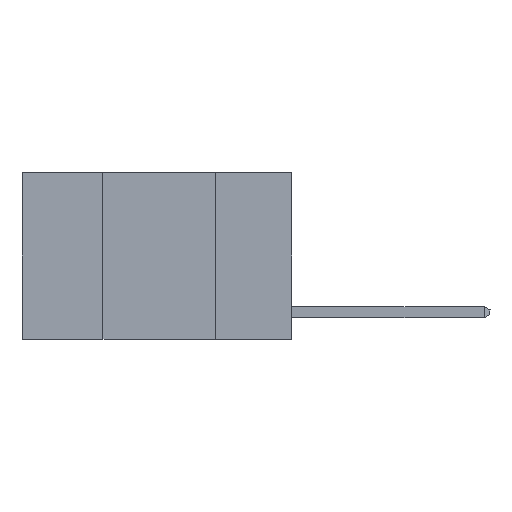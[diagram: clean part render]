
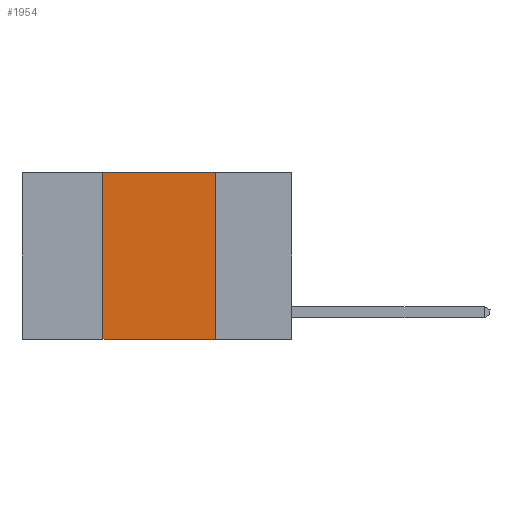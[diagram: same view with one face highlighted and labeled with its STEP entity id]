
A CAD part, left-side view. The second image highlights one B-rep face of the part: STEP entity #1954.
In plain terms, the highlighted planar face has unit normal (-1, 0, 0).
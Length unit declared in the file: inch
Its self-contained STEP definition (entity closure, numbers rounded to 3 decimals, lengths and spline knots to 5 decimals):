
#173 = EDGE_CURVE ( 'NONE', #13643, #10180, #6205, .T. ) ;
#1719 = DIRECTION ( 'NONE',  ( 0., 0., -1. ) ) ;
#1869 = VECTOR ( 'NONE', #1719, 39.37008 ) ;
#1954 = ADVANCED_FACE ( 'NONE', ( #7590 ), #12588, .F. ) ;
#2346 = CARTESIAN_POINT ( 'NONE',  ( 0., 0.42, 0. ) ) ;
#2597 = ORIENTED_EDGE ( 'NONE', *, *, #3217, .T. ) ;
#3217 = EDGE_CURVE ( 'NONE', #7974, #10180, #10415, .T. ) ;
#3267 = DIRECTION ( 'NONE',  ( 0., -1., 0. ) ) ;
#3956 = CARTESIAN_POINT ( 'NONE',  ( 0., 0.42, 0. ) ) ;
#3976 = CARTESIAN_POINT ( 'NONE',  ( 0., 0.6, 0. ) ) ;
#4303 = CARTESIAN_POINT ( 'NONE',  ( 0., 0.42, -0.37 ) ) ;
#5505 = DIRECTION ( 'NONE',  ( 0., -1., 0. ) ) ;
#5755 = CARTESIAN_POINT ( 'NONE',  ( 0., 0.17, -0.37 ) ) ;
#5834 = ORIENTED_EDGE ( 'NONE', *, *, #14758, .F. ) ;
#6205 = LINE ( 'NONE', #9422, #1869 ) ;
#6971 = LINE ( 'NONE', #2346, #10470 ) ;
#7076 = VECTOR ( 'NONE', #5505, 39.37008 ) ;
#7590 = FACE_OUTER_BOUND ( 'NONE', #12613, .T. ) ;
#7974 = VERTEX_POINT ( 'NONE', #4303 ) ;
#8143 = VECTOR ( 'NONE', #3267, 39.37008 ) ;
#8441 = CARTESIAN_POINT ( 'NONE',  ( 0., 0.6, -0.37 ) ) ;
#8486 = DIRECTION ( 'NONE',  ( 0., 0., -1. ) ) ;
#8610 = ORIENTED_EDGE ( 'NONE', *, *, #173, .F. ) ;
#9291 = CARTESIAN_POINT ( 'NONE',  ( 0., 0.17, 0. ) ) ;
#9422 = CARTESIAN_POINT ( 'NONE',  ( 0., 0.17, 0. ) ) ;
#9465 = VERTEX_POINT ( 'NONE', #3956 ) ;
#9805 = CARTESIAN_POINT ( 'NONE',  ( 0., 0.6, 0. ) ) ;
#10180 = VERTEX_POINT ( 'NONE', #5755 ) ;
#10415 = LINE ( 'NONE', #8441, #8143 ) ;
#10470 = VECTOR ( 'NONE', #11625, 39.37008 ) ;
#11370 = LINE ( 'NONE', #3976, #7076 ) ;
#11625 = DIRECTION ( 'NONE',  ( 0., 0., 1. ) ) ;
#12120 = EDGE_CURVE ( 'NONE', #7974, #9465, #6971, .T. ) ;
#12588 = PLANE ( 'NONE',  #15076 ) ;
#12613 = EDGE_LOOP ( 'NONE', ( #8610, #5834, #16317, #2597 ) ) ;
#13643 = VERTEX_POINT ( 'NONE', #9291 ) ;
#14758 = EDGE_CURVE ( 'NONE', #9465, #13643, #11370, .T. ) ;
#15076 = AXIS2_PLACEMENT_3D ( 'NONE', #9805, #16400, #8486 ) ;
#16317 = ORIENTED_EDGE ( 'NONE', *, *, #12120, .F. ) ;
#16400 = DIRECTION ( 'NONE',  ( 1., 0., 0. ) ) ;
